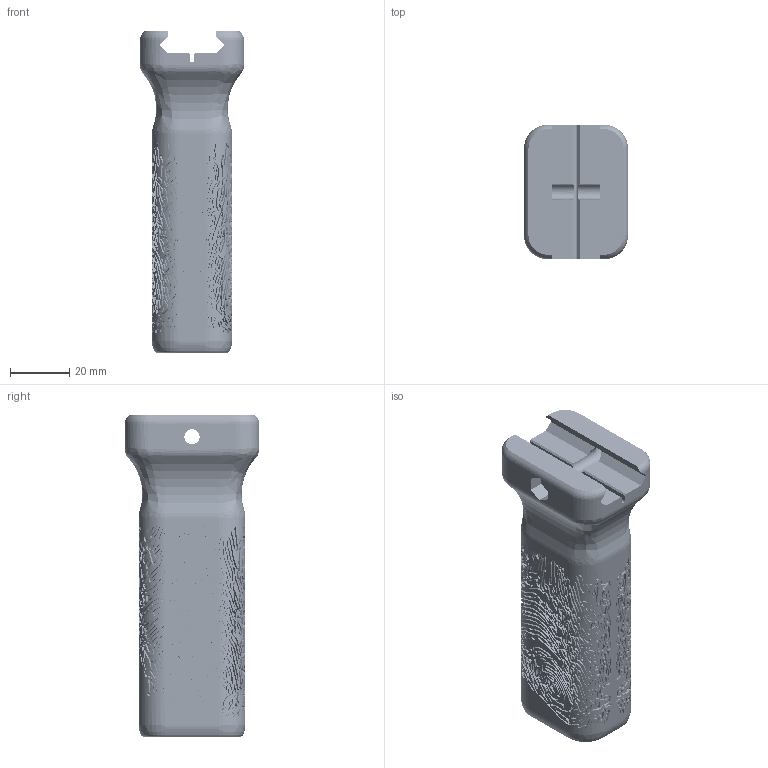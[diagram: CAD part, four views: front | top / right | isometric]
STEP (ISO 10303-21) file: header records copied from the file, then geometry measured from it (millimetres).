
FILE_DESCRIPTION(/* description */ (''),/* implementation_level */ '2;1');
FILE_NAME(/* name */ 'Heretic Model.step',/* time_stamp */ '2021-05-21T12:32:25-04:00',/* author */ (''),/* organization */ (''),/* preprocessor_version */ 'ST-DEVELOPER v18.1',/* originating_system */ 'Autodesk Translation Framework v10.6.0.1341',/* authorisation */ '');
FILE_SCHEMA (('AUTOMOTIVE_DESIGN { 1 0 10303 214 3 1 1 }'));
Products named in the file (1): Heretic Model
Bounding box: 35 x 45.3 x 108.12 mm (x, y, z)
Volume: 54812.9 mm3; surface area: 29503.7 mm2
Topology: 1 solids, 1 shells, 7829 faces, 21195 edges, 13862 vertices
Faces by surface type: bspline 6582, plane 673, cylinder 542, torus 20, cone 12
Full cylindrical faces by diameter (mm): 5.1 x2, 8.75 x1, 11.5 x1, 13 x1
Entity records: 308858 total; most frequent: CARTESIAN_POINT 165974, ORIENTED_EDGE 42382, EDGE_CURVE 21191, VERTEX_POINT 13862, DIRECTION 10823, EDGE_LOOP 8331, FACE_OUTER_BOUND 7829, ADVANCED_FACE 7829
